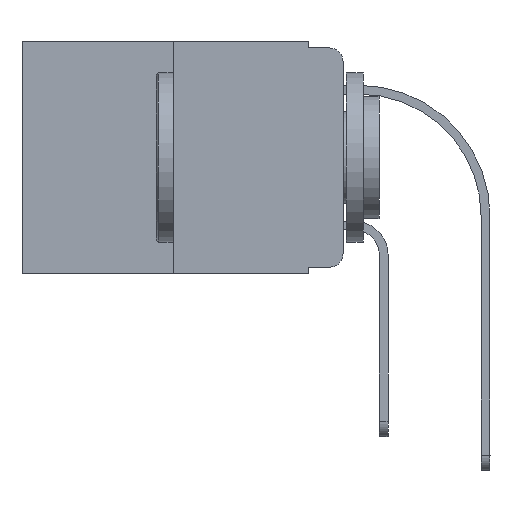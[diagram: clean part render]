
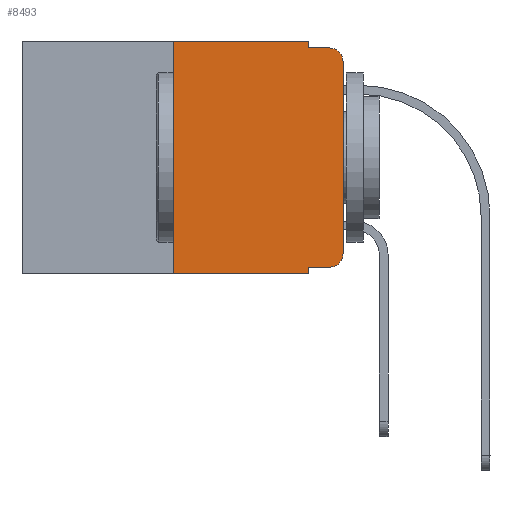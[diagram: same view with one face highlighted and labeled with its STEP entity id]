
A CAD part, left-side view. The second image highlights one B-rep face of the part: STEP entity #8493.
In plain terms, the highlighted planar face has unit normal (-1, 0, 0).
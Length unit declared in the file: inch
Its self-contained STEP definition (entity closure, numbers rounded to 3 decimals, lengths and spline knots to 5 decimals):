
#176 = ORIENTED_EDGE ( 'NONE', *, *, #639, .T. ) ;
#261 = PLANE ( 'NONE',  #5967 ) ;
#344 = DIRECTION ( 'NONE',  ( 0., -1., 0. ) ) ;
#636 = VECTOR ( 'NONE', #3774, 39.37008 ) ;
#639 = EDGE_CURVE ( 'NONE', #2915, #21473, #11340, .T. ) ;
#883 = ORIENTED_EDGE ( 'NONE', *, *, #1868, .F. ) ;
#991 = EDGE_CURVE ( 'NONE', #1627, #15273, #12591, .T. ) ;
#1098 = DIRECTION ( 'NONE',  ( 0., -1., 0. ) ) ;
#1627 = VERTEX_POINT ( 'NONE', #21679 ) ;
#1868 = EDGE_CURVE ( 'NONE', #21986, #2595, #7182, .T. ) ;
#2452 = ORIENTED_EDGE ( 'NONE', *, *, #991, .F. ) ;
#2453 = DIRECTION ( 'NONE',  ( 0., 0., -1. ) ) ;
#2535 = CARTESIAN_POINT ( 'NONE',  ( 0., 0.051, 0. ) ) ;
#2595 = VERTEX_POINT ( 'NONE', #20567 ) ;
#2690 = DIRECTION ( 'NONE',  ( 0., 0., -1. ) ) ;
#2883 = VECTOR ( 'NONE', #12165, 39.37008 ) ;
#2915 = VERTEX_POINT ( 'NONE', #3631 ) ;
#2931 = VECTOR ( 'NONE', #14803, 39.37008 ) ;
#3084 = DIRECTION ( 'NONE',  ( -1., 0., 0. ) ) ;
#3176 = CARTESIAN_POINT ( 'NONE',  ( 0., 0.051, 0. ) ) ;
#3399 = VERTEX_POINT ( 'NONE', #11961 ) ;
#3631 = CARTESIAN_POINT ( 'NONE',  ( 0., 0.02, -0.333 ) ) ;
#3774 = DIRECTION ( 'NONE',  ( 0., -1., 0. ) ) ;
#3905 = CIRCLE ( 'NONE', #16971, 0.02 ) ;
#4203 = CARTESIAN_POINT ( 'NONE',  ( 0., 0.02, -0.313 ) ) ;
#4733 = CARTESIAN_POINT ( 'NONE',  ( 0., 0.051, 0. ) ) ;
#5756 = EDGE_CURVE ( 'NONE', #3399, #13397, #12922, .T. ) ;
#5761 = EDGE_LOOP ( 'NONE', ( #19920, #10517, #883, #23025, #2452, #20350, #8709, #21647, #15245, #176 ) ) ;
#5957 = FACE_OUTER_BOUND ( 'NONE', #5761, .T. ) ;
#5967 = AXIS2_PLACEMENT_3D ( 'NONE', #19736, #17994, #2690 ) ;
#6249 = CARTESIAN_POINT ( 'NONE',  ( 0., 0.02, -0.03 ) ) ;
#7163 = CARTESIAN_POINT ( 'NONE',  ( 0., 0.473, -0.343 ) ) ;
#7182 = LINE ( 'NONE', #12094, #15793 ) ;
#7671 = EDGE_CURVE ( 'NONE', #9440, #2595, #3905, .T. ) ;
#7763 = CARTESIAN_POINT ( 'NONE',  ( 0., 0., 0. ) ) ;
#8021 = CARTESIAN_POINT ( 'NONE',  ( 0., 0., -0.313 ) ) ;
#8101 = EDGE_CURVE ( 'NONE', #3399, #2915, #13453, .T. ) ;
#8493 = ADVANCED_FACE ( 'NONE', ( #5957 ), #261, .F. ) ;
#8615 = DIRECTION ( 'NONE',  ( 0., 0., 1. ) ) ;
#8708 = DIRECTION ( 'NONE',  ( 0., -1., 0. ) ) ;
#8709 = ORIENTED_EDGE ( 'NONE', *, *, #14153, .T. ) ;
#9440 = VERTEX_POINT ( 'NONE', #10076 ) ;
#9746 = CARTESIAN_POINT ( 'NONE',  ( 0., 0.051, -0.01 ) ) ;
#10076 = CARTESIAN_POINT ( 'NONE',  ( 0., 0., -0.03 ) ) ;
#10098 = DIRECTION ( 'NONE',  ( 0., 0., -1. ) ) ;
#10101 = CARTESIAN_POINT ( 'NONE',  ( 0., 0.25, -0.343 ) ) ;
#10517 = ORIENTED_EDGE ( 'NONE', *, *, #7671, .T. ) ;
#10625 = VECTOR ( 'NONE', #21996, 39.37008 ) ;
#11327 = DIRECTION ( 'NONE',  ( -1., 0., 0. ) ) ;
#11340 = CIRCLE ( 'NONE', #12834, 0.02 ) ;
#11961 = CARTESIAN_POINT ( 'NONE',  ( 0., 0.051, -0.333 ) ) ;
#12094 = CARTESIAN_POINT ( 'NONE',  ( 0., 0.051, -0.01 ) ) ;
#12165 = DIRECTION ( 'NONE',  ( 0., 0., -1. ) ) ;
#12532 = LINE ( 'NONE', #7163, #636 ) ;
#12591 = LINE ( 'NONE', #16334, #15647 ) ;
#12834 = AXIS2_PLACEMENT_3D ( 'NONE', #4203, #11327, #2453 ) ;
#12922 = LINE ( 'NONE', #2535, #2931 ) ;
#13397 = VERTEX_POINT ( 'NONE', #22315 ) ;
#13453 = LINE ( 'NONE', #13567, #21273 ) ;
#13567 = CARTESIAN_POINT ( 'NONE',  ( 0., 0.051, -0.333 ) ) ;
#13846 = EDGE_CURVE ( 'NONE', #22680, #1627, #20978, .T. ) ;
#14153 = EDGE_CURVE ( 'NONE', #22680, #13397, #12532, .T. ) ;
#14410 = EDGE_CURVE ( 'NONE', #15273, #21986, #19161, .T. ) ;
#14803 = DIRECTION ( 'NONE',  ( 0., 0., -1. ) ) ;
#15245 = ORIENTED_EDGE ( 'NONE', *, *, #8101, .T. ) ;
#15273 = VERTEX_POINT ( 'NONE', #4733 ) ;
#15647 = VECTOR ( 'NONE', #344, 39.37008 ) ;
#15793 = VECTOR ( 'NONE', #8708, 39.37008 ) ;
#16334 = CARTESIAN_POINT ( 'NONE',  ( 0., 0.473, 0. ) ) ;
#16971 = AXIS2_PLACEMENT_3D ( 'NONE', #6249, #3084, #10098 ) ;
#17405 = VECTOR ( 'NONE', #8615, 39.37008 ) ;
#17994 = DIRECTION ( 'NONE',  ( 1., 0., 0. ) ) ;
#19161 = LINE ( 'NONE', #3176, #2883 ) ;
#19571 = CARTESIAN_POINT ( 'NONE',  ( 0., 0.25, 0. ) ) ;
#19736 = CARTESIAN_POINT ( 'NONE',  ( 0., 0.473, 0. ) ) ;
#19920 = ORIENTED_EDGE ( 'NONE', *, *, #21958, .T. ) ;
#20350 = ORIENTED_EDGE ( 'NONE', *, *, #13846, .F. ) ;
#20367 = LINE ( 'NONE', #7763, #10625 ) ;
#20567 = CARTESIAN_POINT ( 'NONE',  ( 0., 0.02, -0.01 ) ) ;
#20978 = LINE ( 'NONE', #19571, #17405 ) ;
#21273 = VECTOR ( 'NONE', #1098, 39.37008 ) ;
#21473 = VERTEX_POINT ( 'NONE', #8021 ) ;
#21647 = ORIENTED_EDGE ( 'NONE', *, *, #5756, .F. ) ;
#21679 = CARTESIAN_POINT ( 'NONE',  ( 0., 0.25, 0. ) ) ;
#21958 = EDGE_CURVE ( 'NONE', #21473, #9440, #20367, .T. ) ;
#21986 = VERTEX_POINT ( 'NONE', #9746 ) ;
#21996 = DIRECTION ( 'NONE',  ( 0., 0., 1. ) ) ;
#22315 = CARTESIAN_POINT ( 'NONE',  ( 0., 0.051, -0.343 ) ) ;
#22680 = VERTEX_POINT ( 'NONE', #10101 ) ;
#23025 = ORIENTED_EDGE ( 'NONE', *, *, #14410, .F. ) ;
